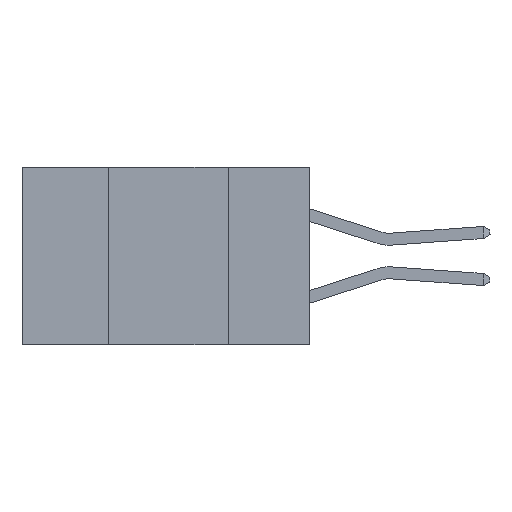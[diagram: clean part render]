
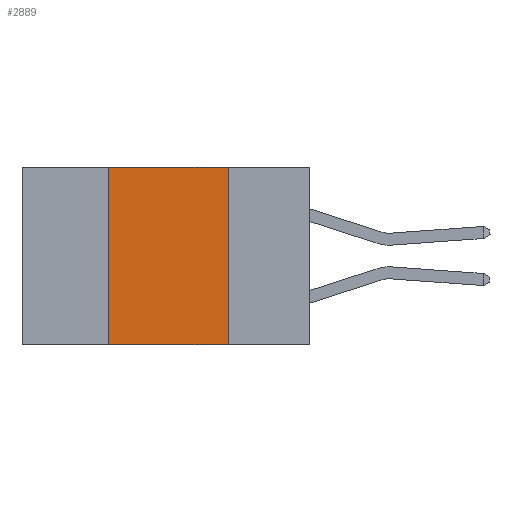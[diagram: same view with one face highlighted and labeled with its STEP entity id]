
A CAD part, left-side view. The second image highlights one B-rep face of the part: STEP entity #2889.
In plain terms, the highlighted planar face has unit normal (-1, 0, 0).
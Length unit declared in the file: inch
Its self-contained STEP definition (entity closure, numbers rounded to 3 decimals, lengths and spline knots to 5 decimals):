
#83 = VERTEX_POINT ( 'NONE', #11126 ) ;
#556 = DIRECTION ( 'NONE',  ( 0., 0., -1. ) ) ;
#651 = EDGE_LOOP ( 'NONE', ( #4798, #2888, #916, #17254 ) ) ;
#864 = CARTESIAN_POINT ( 'NONE',  ( 0., 0.42, 0. ) ) ;
#916 = ORIENTED_EDGE ( 'NONE', *, *, #10342, .F. ) ;
#976 = VERTEX_POINT ( 'NONE', #864 ) ;
#2762 = DIRECTION ( 'NONE',  ( 1., 0., 0. ) ) ;
#2888 = ORIENTED_EDGE ( 'NONE', *, *, #24654, .F. ) ;
#2889 = ADVANCED_FACE ( 'NONE', ( #11244 ), #21675, .F. ) ;
#3574 = CARTESIAN_POINT ( 'NONE',  ( 0., 0.6, -0.37 ) ) ;
#4040 = VECTOR ( 'NONE', #18467, 39.37008 ) ;
#4798 = ORIENTED_EDGE ( 'NONE', *, *, #11273, .F. ) ;
#5771 = LINE ( 'NONE', #26758, #22645 ) ;
#5941 = LINE ( 'NONE', #12347, #4040 ) ;
#10342 = EDGE_CURVE ( 'NONE', #83, #976, #5941, .T. ) ;
#10559 = CARTESIAN_POINT ( 'NONE',  ( 0., 0.17, -0.37 ) ) ;
#11126 = CARTESIAN_POINT ( 'NONE',  ( 0., 0.42, -0.37 ) ) ;
#11244 = FACE_OUTER_BOUND ( 'NONE', #651, .T. ) ;
#11273 = EDGE_CURVE ( 'NONE', #27059, #17975, #19034, .T. ) ;
#11886 = CARTESIAN_POINT ( 'NONE',  ( 0., 0.17, -0.37 ) ) ;
#12055 = DIRECTION ( 'NONE',  ( 0., -1., 0. ) ) ;
#12347 = CARTESIAN_POINT ( 'NONE',  ( 0., 0.42, -0.37 ) ) ;
#12754 = VECTOR ( 'NONE', #12055, 39.37008 ) ;
#13702 = DIRECTION ( 'NONE',  ( 0., -1., 0. ) ) ;
#16136 = AXIS2_PLACEMENT_3D ( 'NONE', #17228, #2762, #556 ) ;
#17228 = CARTESIAN_POINT ( 'NONE',  ( 0., 0.6, 0. ) ) ;
#17254 = ORIENTED_EDGE ( 'NONE', *, *, #21060, .T. ) ;
#17975 = VERTEX_POINT ( 'NONE', #11886 ) ;
#18467 = DIRECTION ( 'NONE',  ( 0., 0., 1. ) ) ;
#19034 = LINE ( 'NONE', #10559, #22311 ) ;
#19797 = CARTESIAN_POINT ( 'NONE',  ( 0., 0.17, 0. ) ) ;
#21060 = EDGE_CURVE ( 'NONE', #83, #17975, #24702, .T. ) ;
#21675 = PLANE ( 'NONE',  #16136 ) ;
#22311 = VECTOR ( 'NONE', #23615, 39.37008 ) ;
#22645 = VECTOR ( 'NONE', #13702, 39.37008 ) ;
#23615 = DIRECTION ( 'NONE',  ( 0., 0., -1. ) ) ;
#24654 = EDGE_CURVE ( 'NONE', #976, #27059, #5771, .T. ) ;
#24702 = LINE ( 'NONE', #3574, #12754 ) ;
#26758 = CARTESIAN_POINT ( 'NONE',  ( 0., 0.6, 0. ) ) ;
#27059 = VERTEX_POINT ( 'NONE', #19797 ) ;
